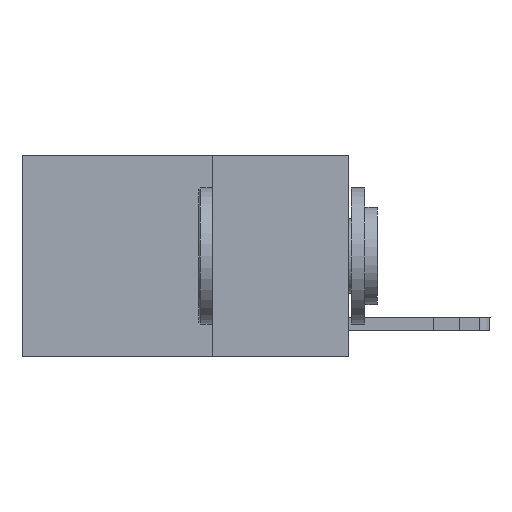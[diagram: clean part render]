
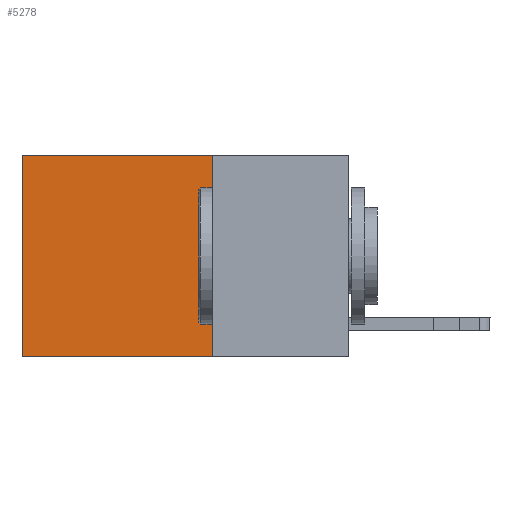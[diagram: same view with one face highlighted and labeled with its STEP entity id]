
A CAD part, left-side view. The second image highlights one B-rep face of the part: STEP entity #5278.
In plain terms, the highlighted planar face has unit normal (-1, 0, 0).
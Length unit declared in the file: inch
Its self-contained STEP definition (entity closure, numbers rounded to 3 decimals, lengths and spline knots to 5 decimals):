
#130 = DIRECTION ( 'NONE',  ( 0., 0., -1. ) ) ;
#236 = DIRECTION ( 'NONE',  ( 1., 0., 0. ) ) ;
#835 = ORIENTED_EDGE ( 'NONE', *, *, #7018, .T. ) ;
#1194 = LINE ( 'NONE', #12975, #6486 ) ;
#1370 = DIRECTION ( 'NONE',  ( 0., 1., 0. ) ) ;
#1383 = VERTEX_POINT ( 'NONE', #13453 ) ;
#1639 = CARTESIAN_POINT ( 'NONE',  ( 0.2625, 0.6, -0.37 ) ) ;
#2177 = ORIENTED_EDGE ( 'NONE', *, *, #11662, .T. ) ;
#3405 = PLANE ( 'NONE',  #3759 ) ;
#3759 = AXIS2_PLACEMENT_3D ( 'NONE', #7711, #236, #8839 ) ;
#3847 = EDGE_CURVE ( 'NONE', #13629, #1383, #1194, .T. ) ;
#5278 = ADVANCED_FACE ( 'NONE', ( #9894 ), #3405, .F. ) ;
#5398 = CARTESIAN_POINT ( 'NONE',  ( 0.2625, 0.6, 0. ) ) ;
#5402 = VECTOR ( 'NONE', #13930, 39.37008 ) ;
#5409 = VECTOR ( 'NONE', #6204, 39.37008 ) ;
#6132 = CARTESIAN_POINT ( 'NONE',  ( 0.2625, 0.25, -0.37 ) ) ;
#6204 = DIRECTION ( 'NONE',  ( 0., 1., 0. ) ) ;
#6486 = VECTOR ( 'NONE', #130, 39.37008 ) ;
#6858 = CARTESIAN_POINT ( 'NONE',  ( 0.2625, 0.25, 0. ) ) ;
#7018 = EDGE_CURVE ( 'NONE', #13534, #9296, #10716, .T. ) ;
#7657 = ORIENTED_EDGE ( 'NONE', *, *, #3847, .F. ) ;
#7711 = CARTESIAN_POINT ( 'NONE',  ( 0.2625, 0.25, 0. ) ) ;
#7821 = EDGE_CURVE ( 'NONE', #1383, #9296, #11466, .T. ) ;
#8839 = DIRECTION ( 'NONE',  ( 0., 0., -1. ) ) ;
#8857 = EDGE_LOOP ( 'NONE', ( #835, #12242, #7657, #2177 ) ) ;
#9057 = LINE ( 'NONE', #13521, #13345 ) ;
#9296 = VERTEX_POINT ( 'NONE', #1639 ) ;
#9757 = CARTESIAN_POINT ( 'NONE',  ( 0.2625, 0.6, 0. ) ) ;
#9894 = FACE_OUTER_BOUND ( 'NONE', #8857, .T. ) ;
#10716 = LINE ( 'NONE', #5398, #5402 ) ;
#11466 = LINE ( 'NONE', #6132, #5409 ) ;
#11662 = EDGE_CURVE ( 'NONE', #13629, #13534, #9057, .T. ) ;
#12242 = ORIENTED_EDGE ( 'NONE', *, *, #7821, .F. ) ;
#12975 = CARTESIAN_POINT ( 'NONE',  ( 0.2625, 0.25, 0. ) ) ;
#13345 = VECTOR ( 'NONE', #1370, 39.37008 ) ;
#13453 = CARTESIAN_POINT ( 'NONE',  ( 0.2625, 0.25, -0.37 ) ) ;
#13521 = CARTESIAN_POINT ( 'NONE',  ( 0.2625, 0.25, 0. ) ) ;
#13534 = VERTEX_POINT ( 'NONE', #9757 ) ;
#13629 = VERTEX_POINT ( 'NONE', #6858 ) ;
#13930 = DIRECTION ( 'NONE',  ( 0., 0., -1. ) ) ;
